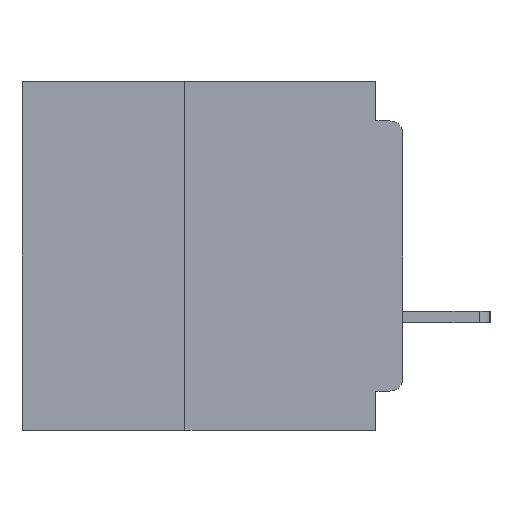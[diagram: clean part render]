
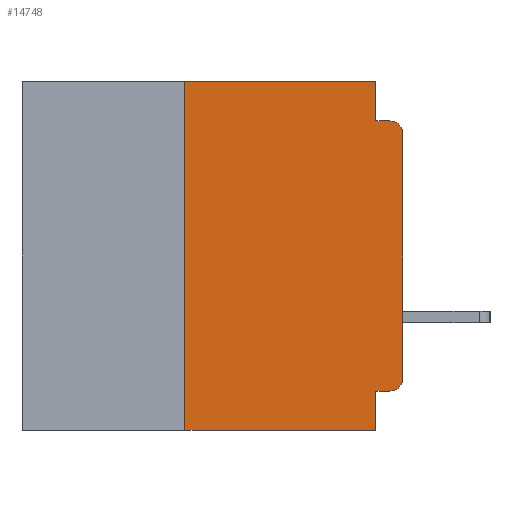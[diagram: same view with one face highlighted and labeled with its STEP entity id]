
A CAD part, left-side view. The second image highlights one B-rep face of the part: STEP entity #14748.
In plain terms, the highlighted planar face has unit normal (-1, 0, 0).
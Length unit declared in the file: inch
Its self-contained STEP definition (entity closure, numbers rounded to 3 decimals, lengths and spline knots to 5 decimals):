
#80 = CARTESIAN_POINT ( 'NONE',  ( 0., 0., -0.355 ) ) ;
#332 = LINE ( 'NONE', #7134, #9626 ) ;
#620 = ORIENTED_EDGE ( 'NONE', *, *, #8175, .F. ) ;
#1915 = EDGE_LOOP ( 'NONE', ( #6842, #19273, #3150, #620, #30635, #29924, #25598, #26485, #45547, #16534 ) ) ;
#2633 = DIRECTION ( 'NONE',  ( 0., -1., 0. ) ) ;
#3150 = ORIENTED_EDGE ( 'NONE', *, *, #8097, .F. ) ;
#3319 = EDGE_CURVE ( 'NONE', #13056, #28766, #39057, .T. ) ;
#3604 = CIRCLE ( 'NONE', #47529, 0.015 ) ;
#3819 = VERTEX_POINT ( 'NONE', #19996 ) ;
#4246 = VERTEX_POINT ( 'NONE', #26380 ) ;
#5046 = VECTOR ( 'NONE', #23493, 39.37008 ) ;
#6075 = CARTESIAN_POINT ( 'NONE',  ( 0., 0.031, -0.355 ) ) ;
#6393 = PLANE ( 'NONE',  #41510 ) ;
#6842 = ORIENTED_EDGE ( 'NONE', *, *, #3319, .T. ) ;
#7134 = CARTESIAN_POINT ( 'NONE',  ( 0., 0.031, -0.4 ) ) ;
#7497 = CARTESIAN_POINT ( 'NONE',  ( 0., 0.015, -0.06 ) ) ;
#8097 = EDGE_CURVE ( 'NONE', #4246, #42532, #14130, .T. ) ;
#8175 = EDGE_CURVE ( 'NONE', #18103, #4246, #41423, .T. ) ;
#9100 = AXIS2_PLACEMENT_3D ( 'NONE', #7497, #34686, #11444 ) ;
#9626 = VECTOR ( 'NONE', #38214, 39.37008 ) ;
#10474 = VECTOR ( 'NONE', #45682, 39.37008 ) ;
#10521 = EDGE_CURVE ( 'NONE', #48811, #13056, #3604, .T. ) ;
#11444 = DIRECTION ( 'NONE',  ( 0., 0., -1. ) ) ;
#12179 = DIRECTION ( 'NONE',  ( 0., -1., 0. ) ) ;
#12187 = VECTOR ( 'NONE', #12179, 39.37008 ) ;
#12357 = FACE_OUTER_BOUND ( 'NONE', #1915, .T. ) ;
#12916 = CARTESIAN_POINT ( 'NONE',  ( 0., 0., 0. ) ) ;
#13056 = VERTEX_POINT ( 'NONE', #48591 ) ;
#13454 = EDGE_CURVE ( 'NONE', #30475, #40120, #41021, .T. ) ;
#14130 = LINE ( 'NONE', #49278, #24431 ) ;
#14275 = DIRECTION ( 'NONE',  ( 1., 0., 0. ) ) ;
#14335 = CARTESIAN_POINT ( 'NONE',  ( 0., 0.25, -0.4 ) ) ;
#14748 = ADVANCED_FACE ( 'NONE', ( #12357 ), #6393, .F. ) ;
#16534 = ORIENTED_EDGE ( 'NONE', *, *, #10521, .T. ) ;
#16560 = CARTESIAN_POINT ( 'NONE',  ( 0., 0.437, -0.4 ) ) ;
#17588 = DIRECTION ( 'NONE',  ( -1., 0., 0. ) ) ;
#17802 = CARTESIAN_POINT ( 'NONE',  ( 0., 0.015, -0.045 ) ) ;
#18103 = VERTEX_POINT ( 'NONE', #45896 ) ;
#19273 = ORIENTED_EDGE ( 'NONE', *, *, #35681, .T. ) ;
#19996 = CARTESIAN_POINT ( 'NONE',  ( 0., 0.031, -0.4 ) ) ;
#21985 = EDGE_CURVE ( 'NONE', #50413, #3819, #332, .T. ) ;
#23493 = DIRECTION ( 'NONE',  ( 0., 1., 0. ) ) ;
#23923 = CARTESIAN_POINT ( 'NONE',  ( 0., 0.25, -0.4 ) ) ;
#24431 = VECTOR ( 'NONE', #2633, 39.37008 ) ;
#24646 = EDGE_CURVE ( 'NONE', #48811, #50413, #33696, .T. ) ;
#24828 = VECTOR ( 'NONE', #39949, 39.37008 ) ;
#25598 = ORIENTED_EDGE ( 'NONE', *, *, #33856, .T. ) ;
#26036 = LINE ( 'NONE', #16560, #24828 ) ;
#26070 = CARTESIAN_POINT ( 'NONE',  ( 0., 0.25, 0. ) ) ;
#26380 = CARTESIAN_POINT ( 'NONE',  ( 0., 0.031, -0.045 ) ) ;
#26485 = ORIENTED_EDGE ( 'NONE', *, *, #21985, .F. ) ;
#26903 = EDGE_CURVE ( 'NONE', #40120, #18103, #44329, .T. ) ;
#27580 = CARTESIAN_POINT ( 'NONE',  ( 0., 0.437, 0. ) ) ;
#27818 = DIRECTION ( 'NONE',  ( 0., 0., 1. ) ) ;
#28766 = VERTEX_POINT ( 'NONE', #29893 ) ;
#29893 = CARTESIAN_POINT ( 'NONE',  ( 0., 0., -0.06 ) ) ;
#29924 = ORIENTED_EDGE ( 'NONE', *, *, #13454, .F. ) ;
#30475 = VERTEX_POINT ( 'NONE', #14335 ) ;
#30635 = ORIENTED_EDGE ( 'NONE', *, *, #26903, .F. ) ;
#30656 = VECTOR ( 'NONE', #27818, 39.37008 ) ;
#32230 = DIRECTION ( 'NONE',  ( 0., 0., 1. ) ) ;
#33696 = LINE ( 'NONE', #80, #5046 ) ;
#33856 = EDGE_CURVE ( 'NONE', #30475, #3819, #26036, .T. ) ;
#34011 = CARTESIAN_POINT ( 'NONE',  ( 0., 0.031, 0. ) ) ;
#34663 = CARTESIAN_POINT ( 'NONE',  ( 0., 0.015, -0.355 ) ) ;
#34686 = DIRECTION ( 'NONE',  ( -1., 0., 0. ) ) ;
#35681 = EDGE_CURVE ( 'NONE', #28766, #42532, #41104, .T. ) ;
#37525 = CARTESIAN_POINT ( 'NONE',  ( 0., 0.437, 0. ) ) ;
#38214 = DIRECTION ( 'NONE',  ( 0., 0., -1. ) ) ;
#39057 = LINE ( 'NONE', #12916, #48157 ) ;
#39949 = DIRECTION ( 'NONE',  ( 0., -1., 0. ) ) ;
#40120 = VERTEX_POINT ( 'NONE', #26070 ) ;
#40808 = CARTESIAN_POINT ( 'NONE',  ( 0., 0.015, -0.34 ) ) ;
#41021 = LINE ( 'NONE', #23923, #30656 ) ;
#41104 = CIRCLE ( 'NONE', #9100, 0.015 ) ;
#41406 = DIRECTION ( 'NONE',  ( 0., 0., -1. ) ) ;
#41423 = LINE ( 'NONE', #34011, #10474 ) ;
#41510 = AXIS2_PLACEMENT_3D ( 'NONE', #37525, #14275, #41406 ) ;
#42532 = VERTEX_POINT ( 'NONE', #17802 ) ;
#44329 = LINE ( 'NONE', #27580, #12187 ) ;
#44696 = DIRECTION ( 'NONE',  ( 0., 0., -1. ) ) ;
#45547 = ORIENTED_EDGE ( 'NONE', *, *, #24646, .F. ) ;
#45682 = DIRECTION ( 'NONE',  ( 0., 0., -1. ) ) ;
#45896 = CARTESIAN_POINT ( 'NONE',  ( 0., 0.031, 0. ) ) ;
#47529 = AXIS2_PLACEMENT_3D ( 'NONE', #40808, #17588, #44696 ) ;
#48157 = VECTOR ( 'NONE', #32230, 39.37008 ) ;
#48591 = CARTESIAN_POINT ( 'NONE',  ( 0., 0., -0.34 ) ) ;
#48811 = VERTEX_POINT ( 'NONE', #34663 ) ;
#49278 = CARTESIAN_POINT ( 'NONE',  ( 0., 0., -0.045 ) ) ;
#50413 = VERTEX_POINT ( 'NONE', #6075 ) ;
